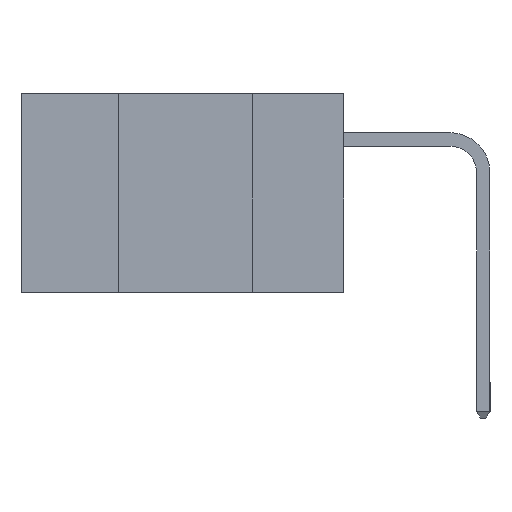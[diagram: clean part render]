
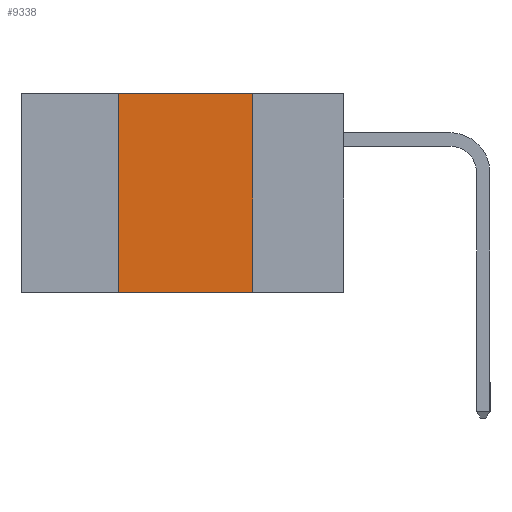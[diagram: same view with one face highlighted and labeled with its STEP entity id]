
A CAD part, left-side view. The second image highlights one B-rep face of the part: STEP entity #9338.
In plain terms, the highlighted planar face has unit normal (-1, 0, 0).
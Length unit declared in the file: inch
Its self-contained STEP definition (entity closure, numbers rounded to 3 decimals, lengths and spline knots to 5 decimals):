
#276 = LINE ( 'NONE', #13855, #22079 ) ;
#3361 = CARTESIAN_POINT ( 'NONE',  ( 0., 0.6, 0. ) ) ;
#5809 = CARTESIAN_POINT ( 'NONE',  ( 0., 0.17, -0.37 ) ) ;
#5988 = DIRECTION ( 'NONE',  ( 0., -1., 0. ) ) ;
#6219 = EDGE_CURVE ( 'NONE', #8849, #23728, #17964, .T. ) ;
#6801 = EDGE_LOOP ( 'NONE', ( #8276, #6899, #9051, #9055 ) ) ;
#6899 = ORIENTED_EDGE ( 'NONE', *, *, #13904, .F. ) ;
#8276 = ORIENTED_EDGE ( 'NONE', *, *, #6219, .F. ) ;
#8786 = CARTESIAN_POINT ( 'NONE',  ( 0., 0.42, 0. ) ) ;
#8849 = VERTEX_POINT ( 'NONE', #13386 ) ;
#9051 = ORIENTED_EDGE ( 'NONE', *, *, #13861, .F. ) ;
#9055 = ORIENTED_EDGE ( 'NONE', *, *, #19012, .T. ) ;
#9338 = ADVANCED_FACE ( 'NONE', ( #12267 ), #23137, .F. ) ;
#9432 = VERTEX_POINT ( 'NONE', #8786 ) ;
#9627 = LINE ( 'NONE', #20533, #21347 ) ;
#10801 = VERTEX_POINT ( 'NONE', #23855 ) ;
#12267 = FACE_OUTER_BOUND ( 'NONE', #6801, .T. ) ;
#12804 = CARTESIAN_POINT ( 'NONE',  ( 0., 0.6, 0. ) ) ;
#13386 = CARTESIAN_POINT ( 'NONE',  ( 0., 0.17, 0. ) ) ;
#13855 = CARTESIAN_POINT ( 'NONE',  ( 0., 0.42, 0. ) ) ;
#13861 = EDGE_CURVE ( 'NONE', #10801, #9432, #276, .T. ) ;
#13904 = EDGE_CURVE ( 'NONE', #9432, #8849, #21424, .T. ) ;
#14958 = DIRECTION ( 'NONE',  ( 0., 0., -1. ) ) ;
#15960 = DIRECTION ( 'NONE',  ( 0., 0., 1. ) ) ;
#16045 = DIRECTION ( 'NONE',  ( 0., -1., 0. ) ) ;
#17964 = LINE ( 'NONE', #23011, #22819 ) ;
#19012 = EDGE_CURVE ( 'NONE', #10801, #23728, #9627, .T. ) ;
#20390 = AXIS2_PLACEMENT_3D ( 'NONE', #12804, #22942, #14958 ) ;
#20533 = CARTESIAN_POINT ( 'NONE',  ( 0., 0.6, -0.37 ) ) ;
#21347 = VECTOR ( 'NONE', #5988, 39.37008 ) ;
#21424 = LINE ( 'NONE', #3361, #26824 ) ;
#22079 = VECTOR ( 'NONE', #15960, 39.37008 ) ;
#22819 = VECTOR ( 'NONE', #25004, 39.37008 ) ;
#22942 = DIRECTION ( 'NONE',  ( 1., 0., 0. ) ) ;
#23011 = CARTESIAN_POINT ( 'NONE',  ( 0., 0.17, 0. ) ) ;
#23137 = PLANE ( 'NONE',  #20390 ) ;
#23728 = VERTEX_POINT ( 'NONE', #5809 ) ;
#23855 = CARTESIAN_POINT ( 'NONE',  ( 0., 0.42, -0.37 ) ) ;
#25004 = DIRECTION ( 'NONE',  ( 0., 0., -1. ) ) ;
#26824 = VECTOR ( 'NONE', #16045, 39.37008 ) ;
